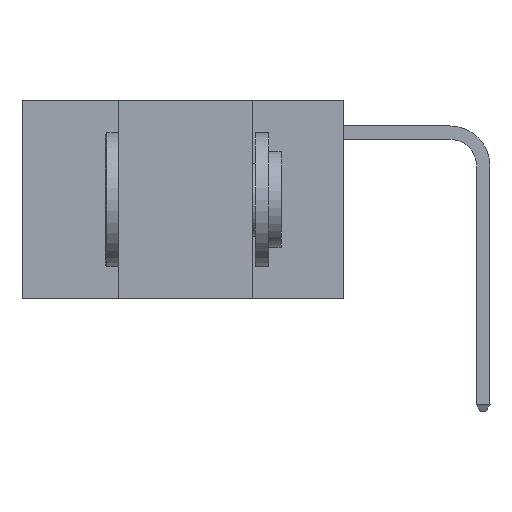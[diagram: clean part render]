
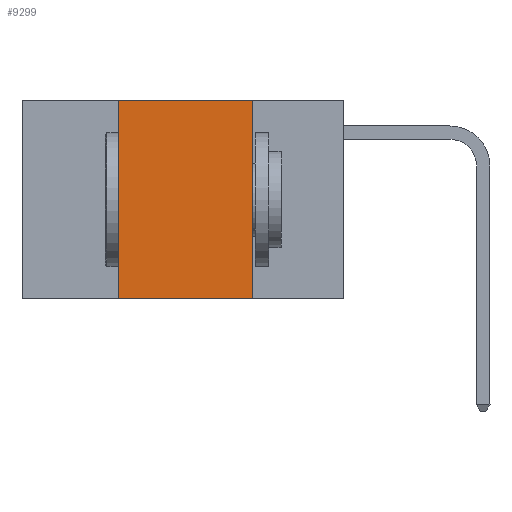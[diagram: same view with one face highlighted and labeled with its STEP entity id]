
A CAD part, left-side view. The second image highlights one B-rep face of the part: STEP entity #9299.
In plain terms, the highlighted planar face has unit normal (-1, 0, 0).
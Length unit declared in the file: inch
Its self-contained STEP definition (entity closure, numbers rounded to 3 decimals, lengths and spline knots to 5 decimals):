
#3141 = VERTEX_POINT ( 'NONE', #12032 ) ;
#4023 = CARTESIAN_POINT ( 'NONE',  ( 0., 0.17, 0. ) ) ;
#4055 = ORIENTED_EDGE ( 'NONE', *, *, #5781, .F. ) ;
#5060 = EDGE_CURVE ( 'NONE', #14500, #3141, #17130, .T. ) ;
#5407 = LINE ( 'NONE', #12046, #19332 ) ;
#5534 = ORIENTED_EDGE ( 'NONE', *, *, #5060, .T. ) ;
#5781 = EDGE_CURVE ( 'NONE', #17386, #11969, #17856, .T. ) ;
#6727 = AXIS2_PLACEMENT_3D ( 'NONE', #11935, #18703, #8867 ) ;
#7375 = VECTOR ( 'NONE', #8243, 39.37008 ) ;
#8243 = DIRECTION ( 'NONE',  ( 0., -1., 0. ) ) ;
#8769 = PLANE ( 'NONE',  #6727 ) ;
#8867 = DIRECTION ( 'NONE',  ( 0., 0., -1. ) ) ;
#9114 = DIRECTION ( 'NONE',  ( 0., 0., -1. ) ) ;
#9299 = ADVANCED_FACE ( 'NONE', ( #17060 ), #8769, .F. ) ;
#9891 = CARTESIAN_POINT ( 'NONE',  ( 0., 0.42, 0. ) ) ;
#10640 = EDGE_CURVE ( 'NONE', #11969, #3141, #17201, .T. ) ;
#11935 = CARTESIAN_POINT ( 'NONE',  ( 0., 0.6, 0. ) ) ;
#11969 = VERTEX_POINT ( 'NONE', #12288 ) ;
#12031 = ORIENTED_EDGE ( 'NONE', *, *, #12233, .F. ) ;
#12032 = CARTESIAN_POINT ( 'NONE',  ( 0., 0.17, -0.37 ) ) ;
#12046 = CARTESIAN_POINT ( 'NONE',  ( 0., 0.42, 0. ) ) ;
#12233 = EDGE_CURVE ( 'NONE', #14500, #17386, #5407, .T. ) ;
#12288 = CARTESIAN_POINT ( 'NONE',  ( 0., 0.17, 0. ) ) ;
#12332 = EDGE_LOOP ( 'NONE', ( #16774, #4055, #12031, #5534 ) ) ;
#13228 = VECTOR ( 'NONE', #9114, 39.37008 ) ;
#14500 = VERTEX_POINT ( 'NONE', #20371 ) ;
#16531 = CARTESIAN_POINT ( 'NONE',  ( 0., 0.6, 0. ) ) ;
#16774 = ORIENTED_EDGE ( 'NONE', *, *, #10640, .F. ) ;
#17060 = FACE_OUTER_BOUND ( 'NONE', #12332, .T. ) ;
#17130 = LINE ( 'NONE', #17230, #21310 ) ;
#17201 = LINE ( 'NONE', #4023, #13228 ) ;
#17230 = CARTESIAN_POINT ( 'NONE',  ( 0., 0.6, -0.37 ) ) ;
#17386 = VERTEX_POINT ( 'NONE', #9891 ) ;
#17856 = LINE ( 'NONE', #16531, #7375 ) ;
#18703 = DIRECTION ( 'NONE',  ( 1., 0., 0. ) ) ;
#18765 = DIRECTION ( 'NONE',  ( 0., -1., 0. ) ) ;
#19259 = DIRECTION ( 'NONE',  ( 0., 0., 1. ) ) ;
#19332 = VECTOR ( 'NONE', #19259, 39.37008 ) ;
#20371 = CARTESIAN_POINT ( 'NONE',  ( 0., 0.42, -0.37 ) ) ;
#21310 = VECTOR ( 'NONE', #18765, 39.37008 ) ;
